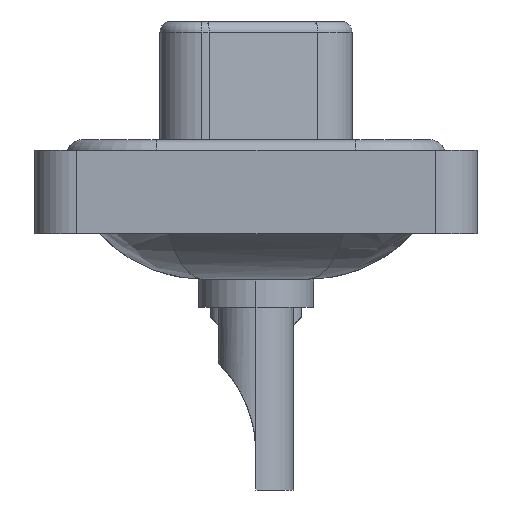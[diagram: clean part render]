
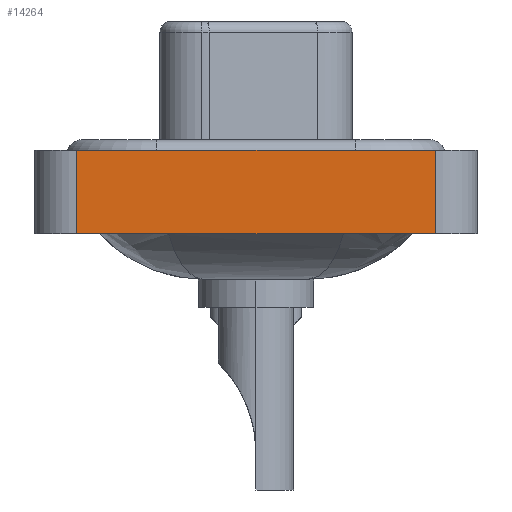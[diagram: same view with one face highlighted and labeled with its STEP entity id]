
A CAD part, left-side view. The second image highlights one B-rep face of the part: STEP entity #14264.
In plain terms, the highlighted planar face has unit normal (-1, 0, 0).
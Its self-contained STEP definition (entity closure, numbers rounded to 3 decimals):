
#6 = VERTEX_POINT ( 'NONE', #16136 ) ;
#504 = DIRECTION ( 'NONE',  ( 0., 0., 1. ) ) ;
#780 = CARTESIAN_POINT ( 'NONE',  ( -7.35, -8.55, 0.4 ) ) ;
#781 = ORIENTED_EDGE ( 'NONE', *, *, #6257, .T. ) ;
#896 = CARTESIAN_POINT ( 'NONE',  ( -7.35, -8.55, -3.6 ) ) ;
#1723 = VERTEX_POINT ( 'NONE', #780 ) ;
#2292 = ORIENTED_EDGE ( 'NONE', *, *, #13627, .T. ) ;
#2687 = LINE ( 'NONE', #896, #18044 ) ;
#4054 = VERTEX_POINT ( 'NONE', #18411 ) ;
#5042 = FACE_OUTER_BOUND ( 'NONE', #6109, .T. ) ;
#5388 = EDGE_CURVE ( 'NONE', #6, #1723, #8821, .T. ) ;
#5877 = ORIENTED_EDGE ( 'NONE', *, *, #5388, .F. ) ;
#6109 = EDGE_LOOP ( 'NONE', ( #781, #5877, #10511, #2292 ) ) ;
#6257 = EDGE_CURVE ( 'NONE', #14078, #1723, #2687, .T. ) ;
#6728 = DIRECTION ( 'NONE',  ( -1., 0., 0. ) ) ;
#7999 = VECTOR ( 'NONE', #504, 1000. ) ;
#8205 = DIRECTION ( 'NONE',  ( 0., 0., 1. ) ) ;
#8821 = LINE ( 'NONE', #14247, #11194 ) ;
#9290 = AXIS2_PLACEMENT_3D ( 'NONE', #12029, #6728, #21224 ) ;
#9633 = VECTOR ( 'NONE', #11473, 1000. ) ;
#10511 = ORIENTED_EDGE ( 'NONE', *, *, #10837, .F. ) ;
#10837 = EDGE_CURVE ( 'NONE', #4054, #6, #19070, .T. ) ;
#10934 = CARTESIAN_POINT ( 'NONE',  ( -7.35, -8.55, -3.6 ) ) ;
#11194 = VECTOR ( 'NONE', #16156, 1000. ) ;
#11473 = DIRECTION ( 'NONE',  ( 0., -1., 0. ) ) ;
#12029 = CARTESIAN_POINT ( 'NONE',  ( -7.35, -8.55, -3.6 ) ) ;
#13627 = EDGE_CURVE ( 'NONE', #4054, #14078, #20817, .T. ) ;
#14078 = VERTEX_POINT ( 'NONE', #10934 ) ;
#14247 = CARTESIAN_POINT ( 'NONE',  ( -7.35, -8.55, 0.4 ) ) ;
#14264 = ADVANCED_FACE ( 'NONE', ( #5042 ), #21557, .T. ) ;
#16136 = CARTESIAN_POINT ( 'NONE',  ( -7.35, 8.55, 0.4 ) ) ;
#16156 = DIRECTION ( 'NONE',  ( 0., -1., 0. ) ) ;
#18044 = VECTOR ( 'NONE', #8205, 1000. ) ;
#18411 = CARTESIAN_POINT ( 'NONE',  ( -7.35, 8.55, -3.6 ) ) ;
#19070 = LINE ( 'NONE', #22159, #7999 ) ;
#20687 = CARTESIAN_POINT ( 'NONE',  ( -7.35, -8.55, -3.6 ) ) ;
#20817 = LINE ( 'NONE', #20687, #9633 ) ;
#21224 = DIRECTION ( 'NONE',  ( 0., 0., 1. ) ) ;
#21557 = PLANE ( 'NONE',  #9290 ) ;
#22159 = CARTESIAN_POINT ( 'NONE',  ( -7.35, 8.55, -3.6 ) ) ;
